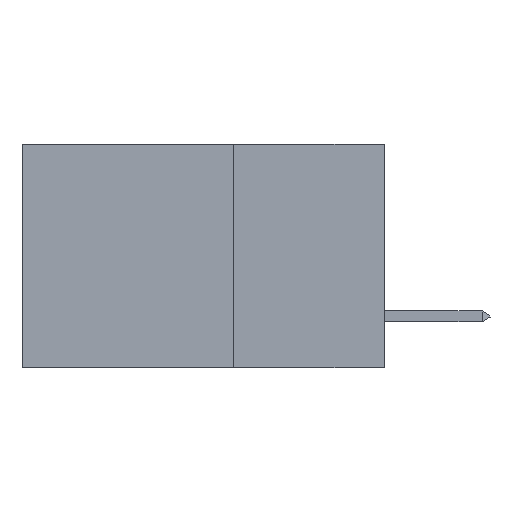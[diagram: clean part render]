
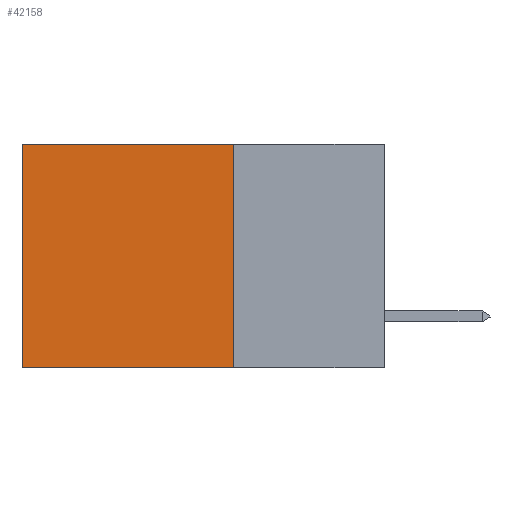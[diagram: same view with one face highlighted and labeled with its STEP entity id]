
A CAD part, left-side view. The second image highlights one B-rep face of the part: STEP entity #42158.
In plain terms, the highlighted planar face has unit normal (-1, 0, 0).
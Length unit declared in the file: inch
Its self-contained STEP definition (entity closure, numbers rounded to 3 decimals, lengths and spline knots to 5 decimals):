
#728 = EDGE_CURVE ( 'NONE', #26355, #25176, #45150, .T. ) ;
#3280 = PLANE ( 'NONE',  #28389 ) ;
#6512 = DIRECTION ( 'NONE',  ( 0., 0., -1. ) ) ;
#6870 = CARTESIAN_POINT ( 'NONE',  ( 0.2875, 0.25, 0. ) ) ;
#7385 = ORIENTED_EDGE ( 'NONE', *, *, #728, .F. ) ;
#9544 = CARTESIAN_POINT ( 'NONE',  ( 0.2875, 0.25, 0. ) ) ;
#12655 = LINE ( 'NONE', #47234, #47839 ) ;
#14395 = FACE_OUTER_BOUND ( 'NONE', #16600, .T. ) ;
#14574 = VECTOR ( 'NONE', #35854, 39.37008 ) ;
#15043 = LINE ( 'NONE', #40628, #26555 ) ;
#16600 = EDGE_LOOP ( 'NONE', ( #34942, #48694, #7385, #40195 ) ) ;
#16848 = CARTESIAN_POINT ( 'NONE',  ( 0.2875, 0.6, 0. ) ) ;
#18137 = CARTESIAN_POINT ( 'NONE',  ( 0.2875, 0.25, 0. ) ) ;
#22799 = CARTESIAN_POINT ( 'NONE',  ( 0.2875, 0.6, -0.37 ) ) ;
#24449 = VECTOR ( 'NONE', #33876, 39.37008 ) ;
#25176 = VERTEX_POINT ( 'NONE', #35152 ) ;
#25925 = DIRECTION ( 'NONE',  ( 1., 0., 0. ) ) ;
#26355 = VERTEX_POINT ( 'NONE', #9544 ) ;
#26555 = VECTOR ( 'NONE', #48282, 39.37008 ) ;
#27022 = EDGE_CURVE ( 'NONE', #26355, #43139, #12655, .T. ) ;
#27608 = CARTESIAN_POINT ( 'NONE',  ( 0.2875, 0.25, -0.37 ) ) ;
#28389 = AXIS2_PLACEMENT_3D ( 'NONE', #18137, #25925, #6512 ) ;
#33315 = VERTEX_POINT ( 'NONE', #22799 ) ;
#33876 = DIRECTION ( 'NONE',  ( 0., 0., -1. ) ) ;
#34942 = ORIENTED_EDGE ( 'NONE', *, *, #40613, .T. ) ;
#34947 = DIRECTION ( 'NONE',  ( 0., 1., 0. ) ) ;
#35152 = CARTESIAN_POINT ( 'NONE',  ( 0.2875, 0.25, -0.37 ) ) ;
#35854 = DIRECTION ( 'NONE',  ( 0., 1., 0. ) ) ;
#39372 = LINE ( 'NONE', #27608, #14574 ) ;
#40195 = ORIENTED_EDGE ( 'NONE', *, *, #27022, .T. ) ;
#40613 = EDGE_CURVE ( 'NONE', #43139, #33315, #15043, .T. ) ;
#40628 = CARTESIAN_POINT ( 'NONE',  ( 0.2875, 0.6, 0. ) ) ;
#42158 = ADVANCED_FACE ( 'NONE', ( #14395 ), #3280, .F. ) ;
#43139 = VERTEX_POINT ( 'NONE', #16848 ) ;
#45150 = LINE ( 'NONE', #6870, #24449 ) ;
#47234 = CARTESIAN_POINT ( 'NONE',  ( 0.2875, 0.25, 0. ) ) ;
#47759 = EDGE_CURVE ( 'NONE', #25176, #33315, #39372, .T. ) ;
#47839 = VECTOR ( 'NONE', #34947, 39.37008 ) ;
#48282 = DIRECTION ( 'NONE',  ( 0., 0., -1. ) ) ;
#48694 = ORIENTED_EDGE ( 'NONE', *, *, #47759, .F. ) ;
